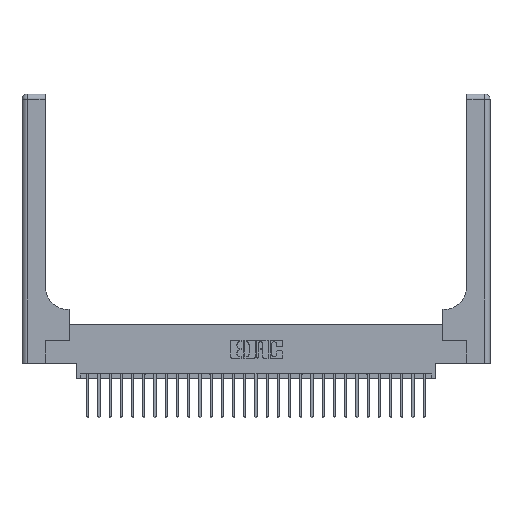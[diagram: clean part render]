
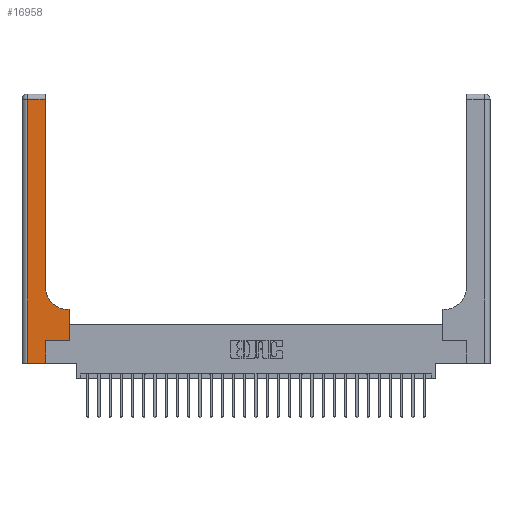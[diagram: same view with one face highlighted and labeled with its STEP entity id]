
A CAD part, top view. The second image highlights one B-rep face of the part: STEP entity #16958.
In plain terms, the highlighted planar face has unit normal (0, 0, 1).
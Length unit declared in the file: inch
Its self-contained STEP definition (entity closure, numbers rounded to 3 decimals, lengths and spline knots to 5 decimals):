
#50 = DIRECTION ( 'NONE',  ( -1., 0., 0. ) ) ;
#68 = CARTESIAN_POINT ( 'NONE',  ( 0.26, 0.6, 0.37 ) ) ;
#373 = CARTESIAN_POINT ( 'NONE',  ( 0.265, 0.25, 0.37 ) ) ;
#651 = CARTESIAN_POINT ( 'NONE',  ( 0.528, 0.6, 0.37 ) ) ;
#1405 = CARTESIAN_POINT ( 'NONE',  ( 0.265, 0.25, 0.37 ) ) ;
#2123 = EDGE_CURVE ( 'NONE', #12319, #5893, #19768, .T. ) ;
#3645 = LINE ( 'NONE', #373, #25266 ) ;
#3686 = VERTEX_POINT ( 'NONE', #24341 ) ;
#4485 = CARTESIAN_POINT ( 'NONE',  ( 0., 2.94, 0.37 ) ) ;
#4734 = ORIENTED_EDGE ( 'NONE', *, *, #13618, .T. ) ;
#5046 = VECTOR ( 'NONE', #25896, 39.37008 ) ;
#5479 = DIRECTION ( 'NONE',  ( 0., 1., 0. ) ) ;
#5514 = VECTOR ( 'NONE', #5479, 39.37008 ) ;
#5893 = VERTEX_POINT ( 'NONE', #15333 ) ;
#6118 = LINE ( 'NONE', #21144, #21612 ) ;
#6294 = EDGE_CURVE ( 'NONE', #20747, #11931, #10984, .T. ) ;
#6364 = DIRECTION ( 'NONE',  ( 0., 1., 0. ) ) ;
#7342 = CARTESIAN_POINT ( 'NONE',  ( 0.06, 2.94, 0.37 ) ) ;
#7620 = LINE ( 'NONE', #17454, #18207 ) ;
#7642 = ORIENTED_EDGE ( 'NONE', *, *, #9987, .T. ) ;
#7963 = ORIENTED_EDGE ( 'NONE', *, *, #22510, .T. ) ;
#8399 = PLANE ( 'NONE',  #24304 ) ;
#8446 = EDGE_LOOP ( 'NONE', ( #4734, #7963, #22669, #9783, #25578, #7642, #18701, #23492, #13261 ) ) ;
#8493 = LINE ( 'NONE', #4485, #18413 ) ;
#9105 = CARTESIAN_POINT ( 'NONE',  ( 0.51, 0.85, 0.37 ) ) ;
#9361 = CARTESIAN_POINT ( 'NONE',  ( 0.265, 0., 0.37 ) ) ;
#9697 = AXIS2_PLACEMENT_3D ( 'NONE', #9105, #23785, #11233 ) ;
#9783 = ORIENTED_EDGE ( 'NONE', *, *, #25422, .T. ) ;
#9987 = EDGE_CURVE ( 'NONE', #11931, #15270, #3645, .T. ) ;
#10142 = CARTESIAN_POINT ( 'NONE',  ( 0.265, 0., 0.37 ) ) ;
#10234 = VERTEX_POINT ( 'NONE', #7342 ) ;
#10984 = LINE ( 'NONE', #10142, #11659 ) ;
#11233 = DIRECTION ( 'NONE',  ( 1., 0., 0. ) ) ;
#11659 = VECTOR ( 'NONE', #20648, 39.37008 ) ;
#11931 = VERTEX_POINT ( 'NONE', #1405 ) ;
#12319 = VERTEX_POINT ( 'NONE', #17256 ) ;
#12481 = FACE_OUTER_BOUND ( 'NONE', #8446, .T. ) ;
#12685 = DIRECTION ( 'NONE',  ( 0., 0., -1. ) ) ;
#12793 = LINE ( 'NONE', #68, #23892 ) ;
#12810 = DIRECTION ( 'NONE',  ( -1., 0., 0. ) ) ;
#13261 = ORIENTED_EDGE ( 'NONE', *, *, #2123, .T. ) ;
#13618 = EDGE_CURVE ( 'NONE', #5893, #20194, #6118, .T. ) ;
#13772 = EDGE_CURVE ( 'NONE', #10234, #3686, #7620, .T. ) ;
#14830 = DIRECTION ( 'NONE',  ( -1., 0., 0. ) ) ;
#15270 = VERTEX_POINT ( 'NONE', #23980 ) ;
#15333 = CARTESIAN_POINT ( 'NONE',  ( 0.26, 0.85, 0.37 ) ) ;
#16022 = CARTESIAN_POINT ( 'NONE',  ( 0.528, 0.25, 0.37 ) ) ;
#16840 = CARTESIAN_POINT ( 'NONE',  ( 0., 3., 0.37 ) ) ;
#16958 = ADVANCED_FACE ( 'NONE', ( #12481 ), #8399, .F. ) ;
#17170 = EDGE_CURVE ( 'NONE', #17982, #12319, #12793, .T. ) ;
#17256 = CARTESIAN_POINT ( 'NONE',  ( 0.51, 0.6, 0.37 ) ) ;
#17454 = CARTESIAN_POINT ( 'NONE',  ( 0.06, 3., 0.37 ) ) ;
#17982 = VERTEX_POINT ( 'NONE', #651 ) ;
#18207 = VECTOR ( 'NONE', #19564, 39.37008 ) ;
#18413 = VECTOR ( 'NONE', #12810, 39.37008 ) ;
#18701 = ORIENTED_EDGE ( 'NONE', *, *, #22863, .T. ) ;
#19364 = DIRECTION ( 'NONE',  ( 1., 0., 0. ) ) ;
#19564 = DIRECTION ( 'NONE',  ( 0., -1., 0. ) ) ;
#19768 = CIRCLE ( 'NONE', #9697, 0.25 ) ;
#19990 = CARTESIAN_POINT ( 'NONE',  ( 0.26, 2.94, 0.37 ) ) ;
#20194 = VERTEX_POINT ( 'NONE', #19990 ) ;
#20648 = DIRECTION ( 'NONE',  ( 0., 1., 0. ) ) ;
#20747 = VERTEX_POINT ( 'NONE', #9361 ) ;
#21144 = CARTESIAN_POINT ( 'NONE',  ( 0.26, 3., 0.37 ) ) ;
#21612 = VECTOR ( 'NONE', #6364, 39.37008 ) ;
#21854 = LINE ( 'NONE', #23867, #5046 ) ;
#22510 = EDGE_CURVE ( 'NONE', #20194, #10234, #8493, .T. ) ;
#22669 = ORIENTED_EDGE ( 'NONE', *, *, #13772, .T. ) ;
#22863 = EDGE_CURVE ( 'NONE', #15270, #17982, #22953, .T. ) ;
#22953 = LINE ( 'NONE', #16022, #5514 ) ;
#23492 = ORIENTED_EDGE ( 'NONE', *, *, #17170, .T. ) ;
#23785 = DIRECTION ( 'NONE',  ( 0., 0., -1. ) ) ;
#23867 = CARTESIAN_POINT ( 'NONE',  ( 0., 0., 0.37 ) ) ;
#23892 = VECTOR ( 'NONE', #14830, 39.37008 ) ;
#23980 = CARTESIAN_POINT ( 'NONE',  ( 0.528, 0.25, 0.37 ) ) ;
#24304 = AXIS2_PLACEMENT_3D ( 'NONE', #16840, #12685, #50 ) ;
#24341 = CARTESIAN_POINT ( 'NONE',  ( 0.06, 0., 0.37 ) ) ;
#25266 = VECTOR ( 'NONE', #19364, 39.37008 ) ;
#25422 = EDGE_CURVE ( 'NONE', #3686, #20747, #21854, .T. ) ;
#25578 = ORIENTED_EDGE ( 'NONE', *, *, #6294, .T. ) ;
#25896 = DIRECTION ( 'NONE',  ( 1., 0., 0. ) ) ;
